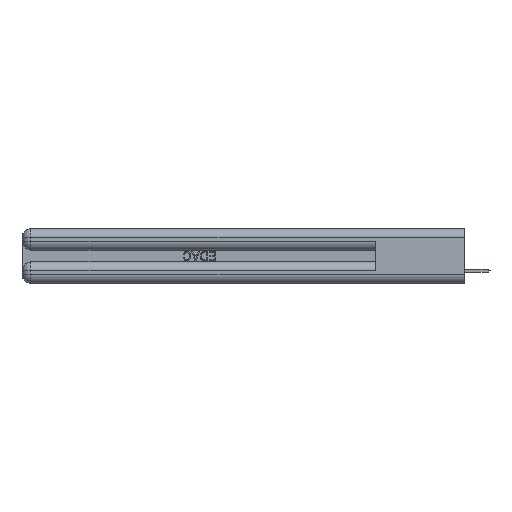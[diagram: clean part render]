
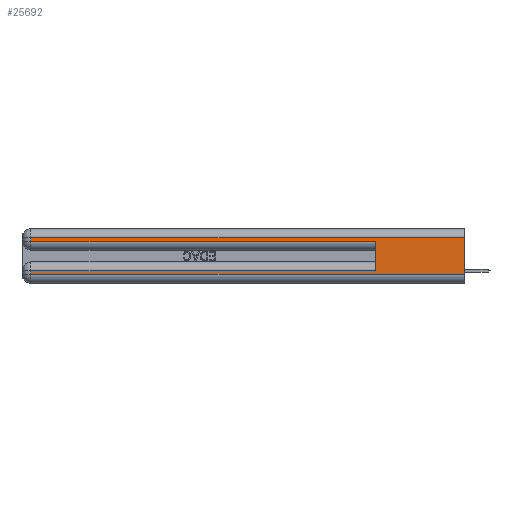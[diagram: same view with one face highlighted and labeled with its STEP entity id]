
A CAD part, left-side view. The second image highlights one B-rep face of the part: STEP entity #25692.
In plain terms, the highlighted planar face has unit normal (-1, 0, 0).
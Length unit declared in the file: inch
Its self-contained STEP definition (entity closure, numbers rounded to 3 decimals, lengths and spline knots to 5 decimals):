
#8 = VECTOR ( 'NONE', #49049, 39.37008 ) ;
#1516 = LINE ( 'NONE', #40575, #35143 ) ;
#1775 = ORIENTED_EDGE ( 'NONE', *, *, #29812, .T. ) ;
#2113 = CARTESIAN_POINT ( 'NONE',  ( 0., 0., 0.06 ) ) ;
#2957 = CARTESIAN_POINT ( 'NONE',  ( 0., 0., 0.31 ) ) ;
#3706 = ORIENTED_EDGE ( 'NONE', *, *, #18401, .T. ) ;
#4120 = AXIS2_PLACEMENT_3D ( 'NONE', #37564, #37904, #34807 ) ;
#7656 = EDGE_CURVE ( 'NONE', #43912, #14238, #35911, .T. ) ;
#8373 = VERTEX_POINT ( 'NONE', #49494 ) ;
#9018 = LINE ( 'NONE', #35229, #28510 ) ;
#9697 = VECTOR ( 'NONE', #38435, 39.37008 ) ;
#12166 = EDGE_CURVE ( 'NONE', #24962, #8373, #41767, .T. ) ;
#13827 = CARTESIAN_POINT ( 'NONE',  ( 0., 2.94, 0.31 ) ) ;
#14238 = VERTEX_POINT ( 'NONE', #48989 ) ;
#14452 = CARTESIAN_POINT ( 'NONE',  ( 0., 2.94, 0.37 ) ) ;
#18401 = EDGE_CURVE ( 'NONE', #24962, #47736, #23903, .T. ) ;
#18554 = DIRECTION ( 'NONE',  ( 0., 0., -1. ) ) ;
#19738 = ORIENTED_EDGE ( 'NONE', *, *, #12166, .F. ) ;
#23232 = LINE ( 'NONE', #14452, #41530 ) ;
#23280 = EDGE_CURVE ( 'NONE', #24776, #29643, #32558, .T. ) ;
#23903 = LINE ( 'NONE', #45921, #33013 ) ;
#24776 = VERTEX_POINT ( 'NONE', #13827 ) ;
#24831 = CARTESIAN_POINT ( 'NONE',  ( 0., 2.94, 0.285 ) ) ;
#24962 = VERTEX_POINT ( 'NONE', #28013 ) ;
#25590 = ORIENTED_EDGE ( 'NONE', *, *, #38176, .F. ) ;
#25692 = ADVANCED_FACE ( 'NONE', ( #29851 ), #33964, .F. ) ;
#28013 = CARTESIAN_POINT ( 'NONE',  ( 0., 0.6, 0.085 ) ) ;
#28510 = VECTOR ( 'NONE', #42931, 39.37008 ) ;
#28873 = ORIENTED_EDGE ( 'NONE', *, *, #35914, .T. ) ;
#29643 = VERTEX_POINT ( 'NONE', #24831 ) ;
#29812 = EDGE_CURVE ( 'NONE', #47736, #43912, #23232, .T. ) ;
#29851 = FACE_OUTER_BOUND ( 'NONE', #39287, .T. ) ;
#30757 = VECTOR ( 'NONE', #45018, 39.37008 ) ;
#31707 = DIRECTION ( 'NONE',  ( 0., 1., 0. ) ) ;
#32110 = DIRECTION ( 'NONE',  ( 0., 0., 1. ) ) ;
#32360 = CARTESIAN_POINT ( 'NONE',  ( 0., 2.94, 0.06 ) ) ;
#32558 = LINE ( 'NONE', #40741, #30757 ) ;
#32640 = CARTESIAN_POINT ( 'NONE',  ( 0., 0.6, 0.145 ) ) ;
#33013 = VECTOR ( 'NONE', #31707, 39.37008 ) ;
#33964 = PLANE ( 'NONE',  #4120 ) ;
#34807 = DIRECTION ( 'NONE',  ( 0., 0., -1. ) ) ;
#35143 = VECTOR ( 'NONE', #36600, 39.37008 ) ;
#35229 = CARTESIAN_POINT ( 'NONE',  ( 0., 0., 0.285 ) ) ;
#35911 = LINE ( 'NONE', #2113, #8 ) ;
#35914 = EDGE_CURVE ( 'NONE', #40873, #24776, #45750, .T. ) ;
#36258 = CARTESIAN_POINT ( 'NONE',  ( 0., 2.94, 0.085 ) ) ;
#36600 = DIRECTION ( 'NONE',  ( 0., 0., -1. ) ) ;
#36670 = EDGE_CURVE ( 'NONE', #29643, #8373, #9018, .T. ) ;
#37564 = CARTESIAN_POINT ( 'NONE',  ( 0., 0., 0.37 ) ) ;
#37787 = ORIENTED_EDGE ( 'NONE', *, *, #23280, .T. ) ;
#37904 = DIRECTION ( 'NONE',  ( 1., 0., 0. ) ) ;
#38176 = EDGE_CURVE ( 'NONE', #40873, #14238, #1516, .T. ) ;
#38435 = DIRECTION ( 'NONE',  ( 0., 1., 0. ) ) ;
#39287 = EDGE_LOOP ( 'NONE', ( #25590, #28873, #37787, #43439, #19738, #3706, #1775, #44278 ) ) ;
#39303 = VECTOR ( 'NONE', #32110, 39.37008 ) ;
#40575 = CARTESIAN_POINT ( 'NONE',  ( 0., 0., 0.37 ) ) ;
#40741 = CARTESIAN_POINT ( 'NONE',  ( 0., 2.94, 0.37 ) ) ;
#40873 = VERTEX_POINT ( 'NONE', #45090 ) ;
#41530 = VECTOR ( 'NONE', #18554, 39.37008 ) ;
#41767 = LINE ( 'NONE', #32640, #39303 ) ;
#42931 = DIRECTION ( 'NONE',  ( 0., -1., 0. ) ) ;
#43439 = ORIENTED_EDGE ( 'NONE', *, *, #36670, .T. ) ;
#43912 = VERTEX_POINT ( 'NONE', #32360 ) ;
#44278 = ORIENTED_EDGE ( 'NONE', *, *, #7656, .T. ) ;
#45018 = DIRECTION ( 'NONE',  ( 0., 0., -1. ) ) ;
#45090 = CARTESIAN_POINT ( 'NONE',  ( 0., 0., 0.31 ) ) ;
#45750 = LINE ( 'NONE', #2957, #9697 ) ;
#45921 = CARTESIAN_POINT ( 'NONE',  ( 0., 0., 0.085 ) ) ;
#47736 = VERTEX_POINT ( 'NONE', #36258 ) ;
#48989 = CARTESIAN_POINT ( 'NONE',  ( 0., 0., 0.06 ) ) ;
#49049 = DIRECTION ( 'NONE',  ( 0., -1., 0. ) ) ;
#49494 = CARTESIAN_POINT ( 'NONE',  ( 0., 0.6, 0.285 ) ) ;
